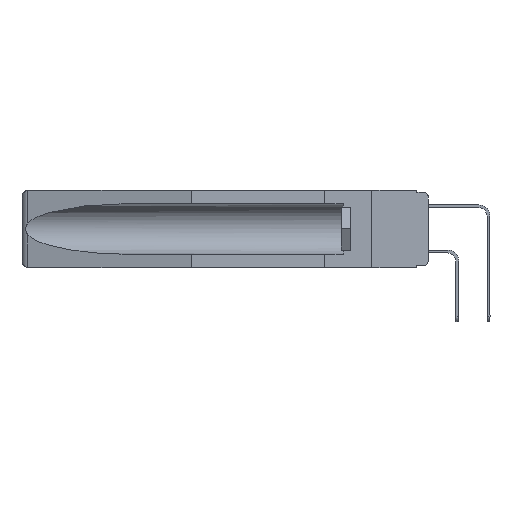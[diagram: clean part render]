
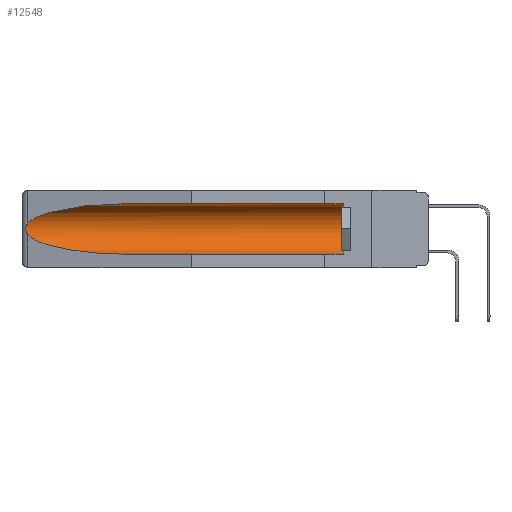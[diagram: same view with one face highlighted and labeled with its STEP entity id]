
A CAD part, left-side view. The second image highlights one B-rep face of the part: STEP entity #12548.
In plain terms, the highlighted cylindrical face has radius 2.857 mm (diameter 5.715 mm), a partial arc.
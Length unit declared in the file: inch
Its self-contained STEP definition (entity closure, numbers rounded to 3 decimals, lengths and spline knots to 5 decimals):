
#322 = EDGE_CURVE ( 'NONE', #20187, #17018, #1101, .T. ) ;
#578 = ORIENTED_EDGE ( 'NONE', *, *, #3383, .T. ) ;
#1101 = LINE ( 'NONE', #12553, #2832 ) ;
#1569 = CARTESIAN_POINT ( 'NONE',  ( 0.21114, 1.30732, -0.059 ) ) ;
#2242 = CARTESIAN_POINT ( 'NONE',  ( 0.26537, 1.52718, -0.19328 ) ) ;
#2260 = DIRECTION ( 'NONE',  ( 0., 1., 0. ) ) ;
#2263 = VECTOR ( 'NONE', #7224, 39.37008 ) ;
#2832 = VECTOR ( 'NONE', #20631, 39.37008 ) ;
#3120 = VERTEX_POINT ( 'NONE', #3182 ) ;
#3182 = CARTESIAN_POINT ( 'NONE',  ( 0.155, 0.126, -0.059 ) ) ;
#3383 = EDGE_CURVE ( 'NONE', #20187, #3120, #5511, .T. ) ;
#3428 = CARTESIAN_POINT ( 'NONE',  ( 0.2675, 1.53308, -0.17534 ) ) ;
#3530 = CARTESIAN_POINT ( 'NONE',  ( 0.26537, 1.52718, -0.14972 ) ) ;
#3575 = FACE_OUTER_BOUND ( 'NONE', #8814, .T. ) ;
#3936 =( BOUNDED_CURVE ( )  B_SPLINE_CURVE ( 3, ( #11979, #10440, #18880, #18567 ),
 .UNSPECIFIED., .F., .T. ) 
 B_SPLINE_CURVE_WITH_KNOTS ( ( 4, 4 ),
 ( 0.1948, 1.5708 ),
 .UNSPECIFIED. ) 
 CURVE ( )  GEOMETRIC_REPRESENTATION_ITEM ( )  RATIONAL_B_SPLINE_CURVE ( ( 1., 0.848, 0.848, 1. ) ) 
 REPRESENTATION_ITEM ( '' )  );
#4598 = ORIENTED_EDGE ( 'NONE', *, *, #18521, .T. ) ;
#5411 = AXIS2_PLACEMENT_3D ( 'NONE', #11768, #2260, #8825 ) ;
#5460 = CARTESIAN_POINT ( 'NONE',  ( 0.26655, 1.53094, -0.18657 ) ) ;
#5511 = CIRCLE ( 'NONE', #7914, 0.1125 ) ;
#6081 = EDGE_CURVE ( 'NONE', #11672, #18480, #7525, .T. ) ;
#6801 = LINE ( 'NONE', #13402, #2263 ) ;
#7224 = DIRECTION ( 'NONE',  ( 0., 1., 0. ) ) ;
#7525 =( BOUNDED_CURVE ( )  B_SPLINE_CURVE ( 3, ( #21222, #1569, #14314, #14430 ),
 .UNSPECIFIED., .F., .T. ) 
 B_SPLINE_CURVE_WITH_KNOTS ( ( 4, 4 ),
 ( 4.71239, 6.08839 ),
 .UNSPECIFIED. ) 
 CURVE ( )  GEOMETRIC_REPRESENTATION_ITEM ( )  RATIONAL_B_SPLINE_CURVE ( ( 1., 0.848, 0.848, 1. ) ) 
 REPRESENTATION_ITEM ( '' )  );
#7914 = AXIS2_PLACEMENT_3D ( 'NONE', #20856, #17625, #20975 ) ;
#8470 = CARTESIAN_POINT ( 'NONE',  ( 0.2675, 1.53308, -0.16763 ) ) ;
#8776 = CARTESIAN_POINT ( 'NONE',  ( 0.26597, 1.5296, -0.19026 ) ) ;
#8814 = EDGE_LOOP ( 'NONE', ( #11911, #4598, #21079, #11136, #578, #13302 ) ) ;
#8825 = DIRECTION ( 'NONE',  ( 0., 0., 1. ) ) ;
#9075 = EDGE_CURVE ( 'NONE', #20791, #17018, #3936, .T. ) ;
#10044 = CARTESIAN_POINT ( 'NONE',  ( 0.155, 0.126, -0.284 ) ) ;
#10440 = CARTESIAN_POINT ( 'NONE',  ( 0.25451, 1.48313, -0.24835 ) ) ;
#11136 = ORIENTED_EDGE ( 'NONE', *, *, #322, .F. ) ;
#11672 = VERTEX_POINT ( 'NONE', #14959 ) ;
#11727 = CARTESIAN_POINT ( 'NONE',  ( 0.26537, 1.52718, -0.14972 ) ) ;
#11768 = CARTESIAN_POINT ( 'NONE',  ( 0.155, -0.30754, -0.1715 ) ) ;
#11806 = CARTESIAN_POINT ( 'NONE',  ( 0.155, 1.07973, -0.284 ) ) ;
#11911 = ORIENTED_EDGE ( 'NONE', *, *, #6081, .T. ) ;
#11979 = CARTESIAN_POINT ( 'NONE',  ( 0.26537, 1.52718, -0.19328 ) ) ;
#12548 = ADVANCED_FACE ( 'NONE', ( #3575 ), #18257, .F. ) ;
#12553 = CARTESIAN_POINT ( 'NONE',  ( 0.155, -0.30754, -0.284 ) ) ;
#13302 = ORIENTED_EDGE ( 'NONE', *, *, #19253, .T. ) ;
#13402 = CARTESIAN_POINT ( 'NONE',  ( 0.155, -0.30754, -0.059 ) ) ;
#14314 = CARTESIAN_POINT ( 'NONE',  ( 0.25451, 1.48313, -0.09465 ) ) ;
#14418 = B_SPLINE_CURVE_WITH_KNOTS ( 'NONE', 3,
 ( #3530, #16685, #20251, #15182, #8470, #3428, #15074, #5460, #8776, #15387 ),
 .UNSPECIFIED., .F., .F.,
 ( 4, 2, 2, 2, 4 ),
 ( 0., 0.00029, 0.00058, 0.00087, 0.00117 ),
 .UNSPECIFIED. ) ;
#14430 = CARTESIAN_POINT ( 'NONE',  ( 0.26537, 1.52718, -0.14972 ) ) ;
#14959 = CARTESIAN_POINT ( 'NONE',  ( 0.155, 1.07973, -0.059 ) ) ;
#15074 = CARTESIAN_POINT ( 'NONE',  ( 0.2673, 1.53269, -0.17917 ) ) ;
#15182 = CARTESIAN_POINT ( 'NONE',  ( 0.2673, 1.5327, -0.16383 ) ) ;
#15387 = CARTESIAN_POINT ( 'NONE',  ( 0.26537, 1.52718, -0.19328 ) ) ;
#16685 = CARTESIAN_POINT ( 'NONE',  ( 0.26597, 1.52961, -0.15275 ) ) ;
#17018 = VERTEX_POINT ( 'NONE', #11806 ) ;
#17625 = DIRECTION ( 'NONE',  ( 0., -1., 0. ) ) ;
#18257 = CYLINDRICAL_SURFACE ( 'NONE', #5411, 0.1125 ) ;
#18480 = VERTEX_POINT ( 'NONE', #11727 ) ;
#18521 = EDGE_CURVE ( 'NONE', #18480, #20791, #14418, .T. ) ;
#18567 = CARTESIAN_POINT ( 'NONE',  ( 0.155, 1.07973, -0.284 ) ) ;
#18880 = CARTESIAN_POINT ( 'NONE',  ( 0.21114, 1.30732, -0.284 ) ) ;
#19253 = EDGE_CURVE ( 'NONE', #3120, #11672, #6801, .T. ) ;
#20187 = VERTEX_POINT ( 'NONE', #10044 ) ;
#20251 = CARTESIAN_POINT ( 'NONE',  ( 0.26654, 1.53092, -0.15636 ) ) ;
#20631 = DIRECTION ( 'NONE',  ( 0., 1., 0. ) ) ;
#20791 = VERTEX_POINT ( 'NONE', #2242 ) ;
#20856 = CARTESIAN_POINT ( 'NONE',  ( 0.155, 0.126, -0.1715 ) ) ;
#20975 = DIRECTION ( 'NONE',  ( 0., 0., 1. ) ) ;
#21079 = ORIENTED_EDGE ( 'NONE', *, *, #9075, .T. ) ;
#21222 = CARTESIAN_POINT ( 'NONE',  ( 0.155, 1.07973, -0.059 ) ) ;
